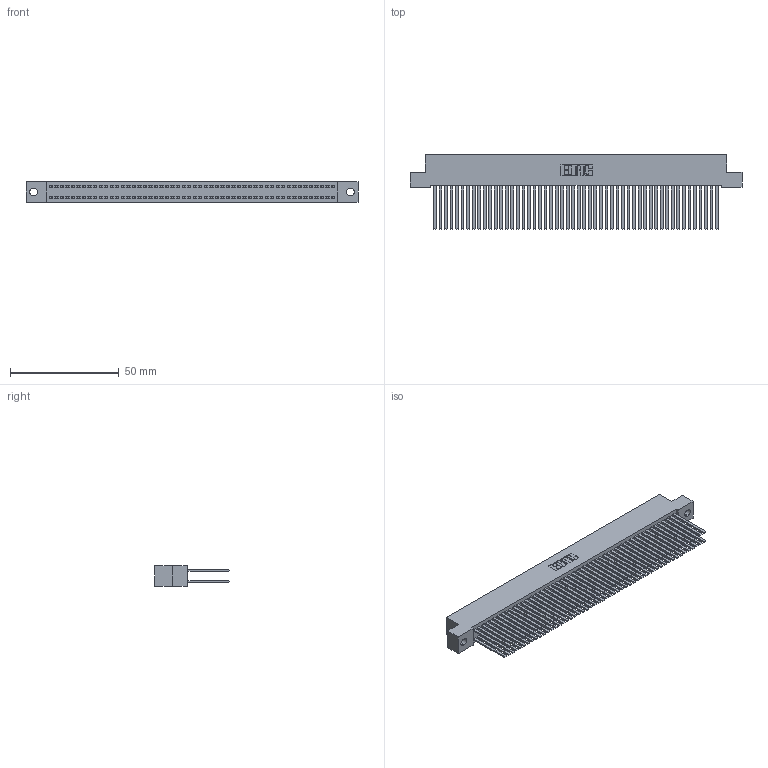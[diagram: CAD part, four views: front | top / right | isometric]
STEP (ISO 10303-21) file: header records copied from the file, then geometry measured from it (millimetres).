
FILE_DESCRIPTION (( 'STEP AP203' ), '1' );
FILE_NAME ('392-104-544-202.STEP', '2018-08-18T19:42:30', ( '' ), ( '' ), 'SwSTEP 2.0', 'SolidWorks 2016', '' );
FILE_SCHEMA (( 'CONFIG_CONTROL_DESIGN' ));
Length unit declared in the file: inch
Products named in the file (3): 342 Part_.128 Slot; 345-292-001_345-293-144; 392-104-544-202
Assembly tree (105 placements, depth 2):
  392-104-544-202
    342 Part_.128 Slot
    345-292-001_345-293-144  x104
Bounding box: 152.4 x 34.3 x 9.4 mm (x, y, z)
Volume: 15146.2 mm3; surface area: 28697.5 mm2
Topology: 105 solids, 105 shells, 4898 faces, 14559 edges, 9566 vertices
Faces by surface type: plane 3398, cylinder 1500
Entity records: 31979 total; most frequent: CARTESIAN_POINT 5286, ORIENTED_EDGE 5222, DIRECTION 4495, EDGE_CURVE 2611, VECTOR 2487, LINE 2487, VERTEX_POINT 1738, AXIS2_PLACEMENT_3D 1004
